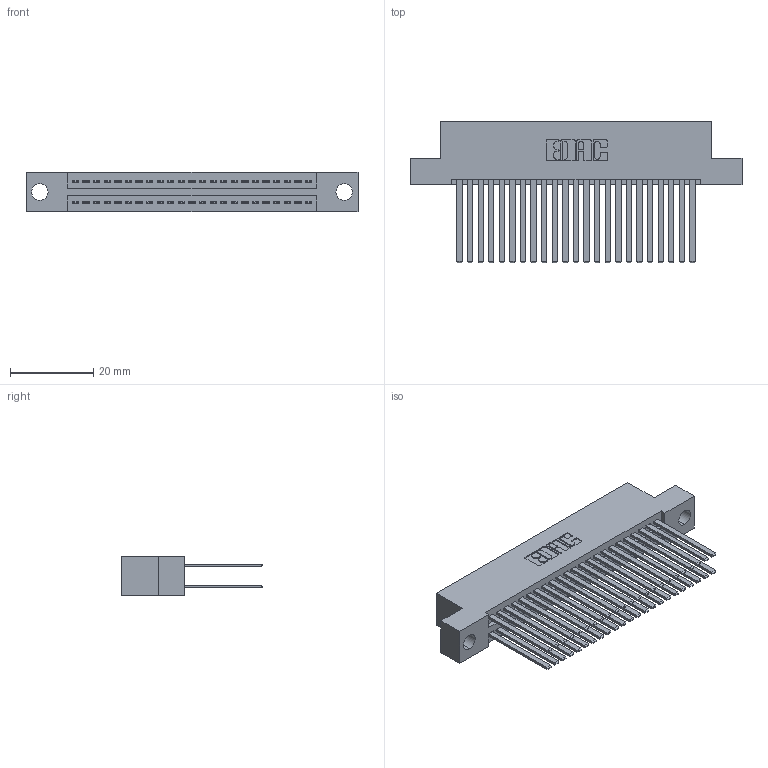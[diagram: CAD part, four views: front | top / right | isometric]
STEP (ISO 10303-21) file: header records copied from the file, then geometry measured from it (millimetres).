
FILE_DESCRIPTION (( 'STEP AP203' ), '1' );
FILE_NAME ('395-046-544-204.STEP', '2021-06-16T23:06:45', ( '' ), ( '' ), 'SwSTEP 2.0', 'SolidWorks 2020', '' );
FILE_SCHEMA (( 'CONFIG_CONTROL_DESIGN' ));
Length unit declared in the file: inch
Products named in the file (3): 345 Part_Flush Mounting Lugs - 0.156 Dia-TI; 345-292-001_345-293-144; 395-046-544-204
Assembly tree (47 placements, depth 2):
  395-046-544-204
    345 Part_Flush Mounting Lugs - 0.156 Dia-TI
    345-292-001_345-293-144  x46
Bounding box: 79.63 x 33.96 x 9.4 mm (x, y, z)
Volume: 8097.8 mm3; surface area: 13343.4 mm2
Topology: 47 solids, 47 shells, 2164 faces, 6403 edges, 4206 vertices
Faces by surface type: plane 1428, cylinder 736
Entity records: 20839 total; most frequent: CARTESIAN_POINT 3514, ORIENTED_EDGE 3446, DIRECTION 3119, EDGE_CURVE 1723, LINE 1503, VECTOR 1503, VERTEX_POINT 1146, AXIS2_PLACEMENT_3D 808
